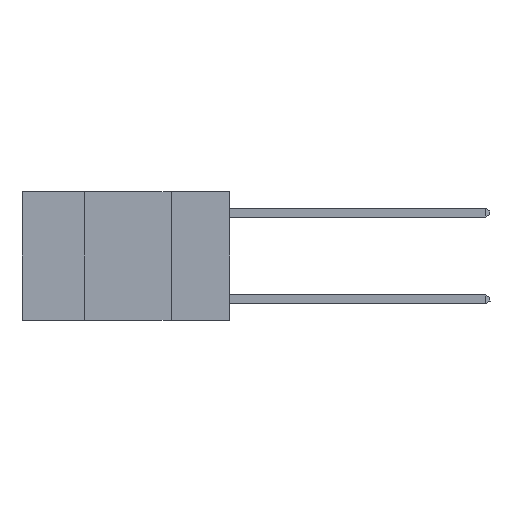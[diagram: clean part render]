
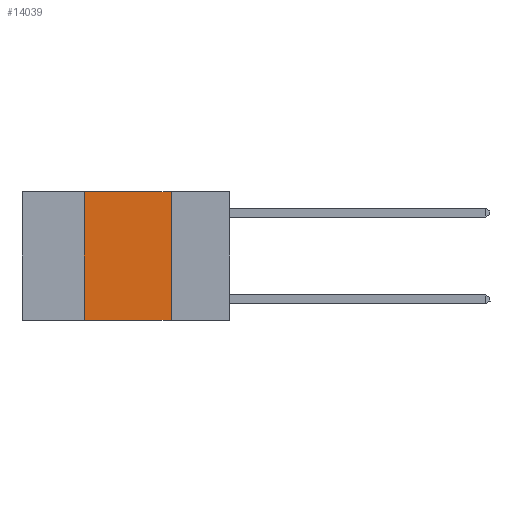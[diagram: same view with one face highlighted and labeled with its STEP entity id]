
A CAD part, left-side view. The second image highlights one B-rep face of the part: STEP entity #14039.
In plain terms, the highlighted planar face has unit normal (-1, 0, 0).
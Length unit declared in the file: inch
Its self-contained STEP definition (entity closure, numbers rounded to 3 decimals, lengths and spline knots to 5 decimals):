
#762 = VERTEX_POINT ( 'NONE', #11294 ) ;
#2097 = CARTESIAN_POINT ( 'NONE',  ( 0., 0.42, 0. ) ) ;
#2244 = ORIENTED_EDGE ( 'NONE', *, *, #13229, .T. ) ;
#3052 = CARTESIAN_POINT ( 'NONE',  ( 0., 0.17, 0. ) ) ;
#3361 = DIRECTION ( 'NONE',  ( 0., -1., 0. ) ) ;
#3509 = CARTESIAN_POINT ( 'NONE',  ( 0., 0.17, -0.37 ) ) ;
#4040 = CARTESIAN_POINT ( 'NONE',  ( 0., 0.6, -0.37 ) ) ;
#5516 = FACE_OUTER_BOUND ( 'NONE', #14265, .T. ) ;
#5689 = VERTEX_POINT ( 'NONE', #3509 ) ;
#6788 = DIRECTION ( 'NONE',  ( 0., 0., 1. ) ) ;
#7807 = CARTESIAN_POINT ( 'NONE',  ( 0., 0.6, 0. ) ) ;
#7897 = LINE ( 'NONE', #3052, #19680 ) ;
#8668 = LINE ( 'NONE', #4040, #16873 ) ;
#9000 = ORIENTED_EDGE ( 'NONE', *, *, #9103, .F. ) ;
#9103 = EDGE_CURVE ( 'NONE', #11892, #5689, #7897, .T. ) ;
#9330 = DIRECTION ( 'NONE',  ( 0., 0., -1. ) ) ;
#9814 = LINE ( 'NONE', #2097, #13917 ) ;
#9859 = EDGE_CURVE ( 'NONE', #762, #11892, #11198, .T. ) ;
#9957 = ORIENTED_EDGE ( 'NONE', *, *, #9859, .F. ) ;
#10812 = PLANE ( 'NONE',  #11629 ) ;
#11024 = CARTESIAN_POINT ( 'NONE',  ( 0., 0.6, 0. ) ) ;
#11198 = LINE ( 'NONE', #11024, #14331 ) ;
#11294 = CARTESIAN_POINT ( 'NONE',  ( 0., 0.42, 0. ) ) ;
#11629 = AXIS2_PLACEMENT_3D ( 'NONE', #7807, #18573, #9330 ) ;
#11892 = VERTEX_POINT ( 'NONE', #17128 ) ;
#12274 = DIRECTION ( 'NONE',  ( 0., 0., -1. ) ) ;
#12540 = VERTEX_POINT ( 'NONE', #15603 ) ;
#13229 = EDGE_CURVE ( 'NONE', #12540, #5689, #8668, .T. ) ;
#13917 = VECTOR ( 'NONE', #6788, 39.37008 ) ;
#14039 = ADVANCED_FACE ( 'NONE', ( #5516 ), #10812, .F. ) ;
#14252 = EDGE_CURVE ( 'NONE', #12540, #762, #9814, .T. ) ;
#14265 = EDGE_LOOP ( 'NONE', ( #9000, #9957, #18177, #2244 ) ) ;
#14331 = VECTOR ( 'NONE', #3361, 39.37008 ) ;
#15603 = CARTESIAN_POINT ( 'NONE',  ( 0., 0.42, -0.37 ) ) ;
#16873 = VECTOR ( 'NONE', #19378, 39.37008 ) ;
#17128 = CARTESIAN_POINT ( 'NONE',  ( 0., 0.17, 0. ) ) ;
#18177 = ORIENTED_EDGE ( 'NONE', *, *, #14252, .F. ) ;
#18573 = DIRECTION ( 'NONE',  ( 1., 0., 0. ) ) ;
#19378 = DIRECTION ( 'NONE',  ( 0., -1., 0. ) ) ;
#19680 = VECTOR ( 'NONE', #12274, 39.37008 ) ;
